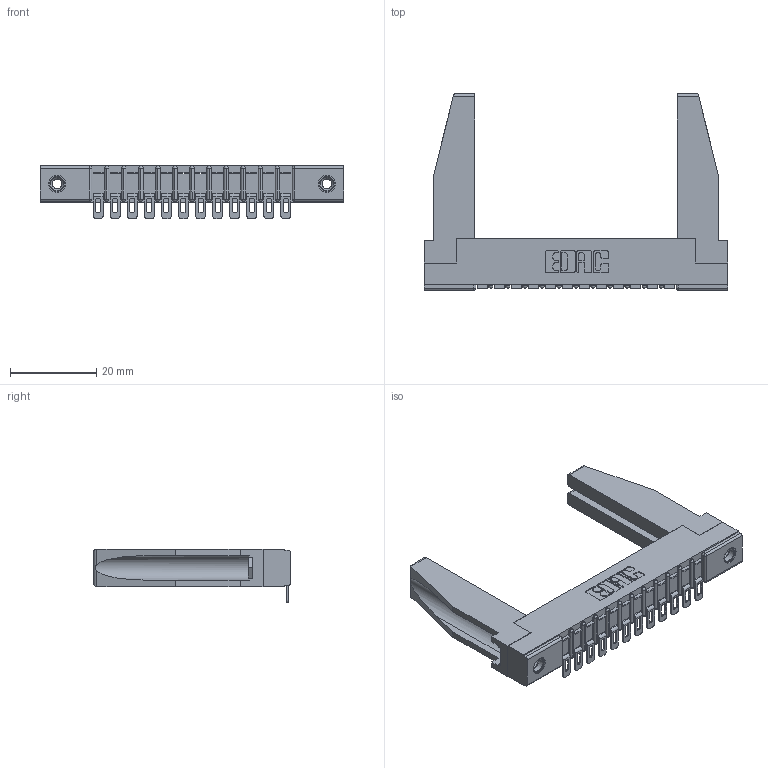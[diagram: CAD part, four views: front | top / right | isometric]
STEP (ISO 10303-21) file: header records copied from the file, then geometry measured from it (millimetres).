
FILE_DESCRIPTION (( 'STEP AP203' ), '1' );
FILE_NAME ('357-012-554-178.STEP', '2019-09-16T19:21:28', ( '' ), ( '' ), 'SwSTEP 2.0', 'SolidWorks 2016', '' );
FILE_SCHEMA (( 'CONFIG_CONTROL_DESIGN' ));
Length unit declared in the file: inch
Products named in the file (5): 345-250-001_345-250-001-102; 307-290-002_554; 307-220-078; 307 Part_.156 Dia Mounting Holes; 357-012-554-178
Assembly tree (17 placements, depth 2):
  357-012-554-178
    307 Part_.156 Dia Mounting Holes
    307-290-002_554  x12
    307-220-078  x2
    345-250-001_345-250-001-102  x2
Bounding box: 70.56 x 45.72 x 12.52 mm (x, y, z)
Volume: 8650.7 mm3; surface area: 11785.1 mm2
Topology: 17 solids, 17 shells, 1233 faces, 3689 edges, 2414 vertices
Faces by surface type: plane 706, cylinder 485, sphere 26, cone 12, torus 4
Entity records: 17390 total; most frequent: CARTESIAN_POINT 2928, ORIENTED_EDGE 2874, DIRECTION 2821, EDGE_CURVE 1437, VECTOR 1083, LINE 1083, VERTEX_POINT 934, AXIS2_PLACEMENT_3D 869
